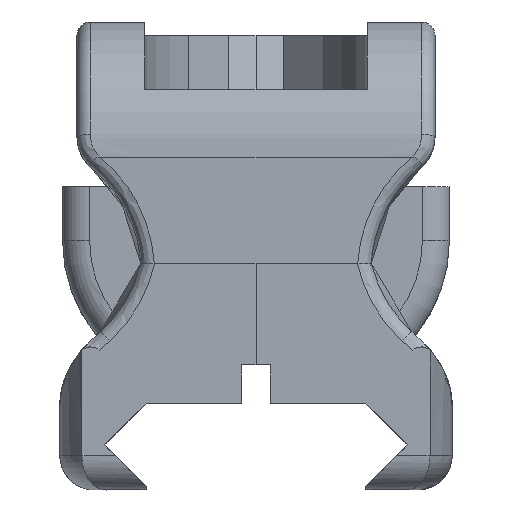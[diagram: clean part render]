
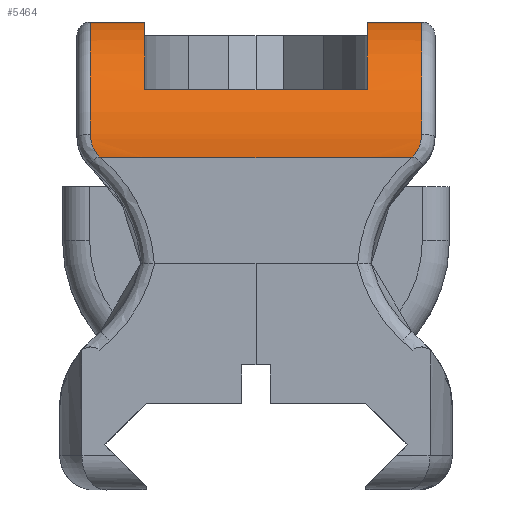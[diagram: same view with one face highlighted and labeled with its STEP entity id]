
A CAD part, front view. The second image highlights one B-rep face of the part: STEP entity #5464.
In plain terms, the highlighted cylindrical face has radius 10 mm (diameter 20 mm), a partial arc.
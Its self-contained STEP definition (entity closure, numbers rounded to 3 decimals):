
#151=B_SPLINE_CURVE_WITH_KNOTS('',3,(#8358,#8359,#8360,#8361,#8362),
 .UNSPECIFIED.,.F.,.F.,(4,1,4),(-0.17,-0.085,0.),
 .UNSPECIFIED.);
#167=B_SPLINE_CURVE_WITH_KNOTS('',3,(#8548,#8549,#8550,#8551,#8552,#8553,
#8554),.UNSPECIFIED.,.F.,.F.,(4,3,4),(-0.004,0.,0.005),
 .UNSPECIFIED.);
#248=B_SPLINE_CURVE_WITH_KNOTS('',3,(#10357,#10358,#10359,#10360,#10361),
 .UNSPECIFIED.,.F.,.F.,(4,1,4),(-0.17,-0.085,0.),
 .UNSPECIFIED.);
#260=B_SPLINE_CURVE_WITH_KNOTS('',3,(#10519,#10520,#10521,#10522,#10523,
#10524,#10525),.UNSPECIFIED.,.F.,.F.,(4,3,4),(-0.004,0.,0.005),
 .UNSPECIFIED.);
#382=CYLINDRICAL_SURFACE('',#5868,10.);
#394=CIRCLE('',#5491,10.);
#396=CIRCLE('',#5495,10.);
#431=CIRCLE('',#5583,10.);
#491=CIRCLE('',#5751,10.);
#522=CIRCLE('',#5866,10.);
#523=CIRCLE('',#5867,10.);
#809=FACE_OUTER_BOUND('',#1103,.T.);
#1103=EDGE_LOOP('',(#4987,#4988,#4989,#4990,#4991,#4992,#4993,#4994,#4995,
#4996,#4997,#4998,#4999,#5000,#5001,#5002));
#1115=LINE('',#7130,#1568);
#1243=LINE('',#8377,#1696);
#1424=LINE('',#10363,#1877);
#1554=LINE('',#11686,#2007);
#1555=LINE('',#11690,#2008);
#1556=LINE('',#11693,#2009);
#1568=VECTOR('',#5890,10.);
#1696=VECTOR('',#6220,10.);
#1877=VECTOR('',#6733,10.);
#2007=VECTOR('',#7089,10.);
#2008=VECTOR('',#7092,10.);
#2009=VECTOR('',#7095,10.);
#2021=VERTEX_POINT('',#7127);
#2022=VERTEX_POINT('',#7129);
#2042=VERTEX_POINT('',#7174);
#2046=VERTEX_POINT('',#7186);
#2208=VERTEX_POINT('',#8306);
#2209=VERTEX_POINT('',#8308);
#2211=VERTEX_POINT('',#8337);
#2226=VERTEX_POINT('',#8542);
#2415=VERTEX_POINT('',#10295);
#2416=VERTEX_POINT('',#10297);
#2418=VERTEX_POINT('',#10326);
#2432=VERTEX_POINT('',#10518);
#2538=VERTEX_POINT('',#11685);
#2539=VERTEX_POINT('',#11687);
#2540=VERTEX_POINT('',#11689);
#2541=VERTEX_POINT('',#11691);
#2552=EDGE_CURVE('',#2021,#2022,#1115,.T.);
#2576=EDGE_CURVE('',#2021,#2042,#394,.T.);
#2581=EDGE_CURVE('',#2022,#2046,#396,.T.);
#2789=EDGE_CURVE('',#2208,#2209,#431,.T.);
#2792=EDGE_CURVE('',#2211,#2208,#151,.T.);
#2797=EDGE_CURVE('',#2209,#2042,#1243,.T.);
#2816=EDGE_CURVE('',#2226,#2211,#167,.T.);
#3133=EDGE_CURVE('',#2415,#2416,#491,.T.);
#3137=EDGE_CURVE('',#2418,#2415,#248,.T.);
#3138=EDGE_CURVE('',#2416,#2046,#1424,.T.);
#3157=EDGE_CURVE('',#2432,#2418,#260,.T.);
#3361=EDGE_CURVE('',#2538,#2432,#1554,.T.);
#3362=EDGE_CURVE('',#2538,#2539,#522,.T.);
#3363=EDGE_CURVE('',#2539,#2540,#1555,.T.);
#3364=EDGE_CURVE('',#2541,#2540,#523,.T.);
#3365=EDGE_CURVE('',#2541,#2226,#1556,.T.);
#4987=ORIENTED_EDGE('',*,*,#3363,.F.);
#4988=ORIENTED_EDGE('',*,*,#3362,.F.);
#4989=ORIENTED_EDGE('',*,*,#3361,.T.);
#4990=ORIENTED_EDGE('',*,*,#3157,.T.);
#4991=ORIENTED_EDGE('',*,*,#3137,.T.);
#4992=ORIENTED_EDGE('',*,*,#3133,.T.);
#4993=ORIENTED_EDGE('',*,*,#3138,.T.);
#4994=ORIENTED_EDGE('',*,*,#2581,.F.);
#4995=ORIENTED_EDGE('',*,*,#2552,.F.);
#4996=ORIENTED_EDGE('',*,*,#2576,.T.);
#4997=ORIENTED_EDGE('',*,*,#2797,.F.);
#4998=ORIENTED_EDGE('',*,*,#2789,.F.);
#4999=ORIENTED_EDGE('',*,*,#2792,.F.);
#5000=ORIENTED_EDGE('',*,*,#2816,.F.);
#5001=ORIENTED_EDGE('',*,*,#3365,.F.);
#5002=ORIENTED_EDGE('',*,*,#3364,.T.);
#5464=ADVANCED_FACE('',(#809),#382,.T.);
#5491=AXIS2_PLACEMENT_3D('',#7176,#5921,#5922);
#5495=AXIS2_PLACEMENT_3D('',#7187,#5932,#5933);
#5583=AXIS2_PLACEMENT_3D('',#8309,#6211,#6212);
#5751=AXIS2_PLACEMENT_3D('',#10299,#6729,#6730);
#5866=AXIS2_PLACEMENT_3D('',#11688,#7090,#7091);
#5867=AXIS2_PLACEMENT_3D('',#11692,#7093,#7094);
#5868=AXIS2_PLACEMENT_3D('',#11694,#7096,#7097);
#5890=DIRECTION('',(1.,0.,0.));
#5921=DIRECTION('center_axis',(-1.,0.,0.));
#5922=DIRECTION('ref_axis',(0.,0.707,0.707));
#5932=DIRECTION('center_axis',(-1.,0.,
0.));
#5933=DIRECTION('ref_axis',(0.,0.707,0.707));
#6211=DIRECTION('center_axis',(-1.,0.,
0.));
#6212=DIRECTION('ref_axis',(0.,-0.804,0.595));
#6220=DIRECTION('',(1.,0.,0.));
#6729=DIRECTION('center_axis',(-1.,0.,
0.));
#6730=DIRECTION('ref_axis',(0.,-0.804,0.595));
#6733=DIRECTION('',(-1.,0.,0.));
#7089=DIRECTION('',(1.,0.,0.));
#7090=DIRECTION('center_axis',(1.,0.,0.));
#7091=DIRECTION('ref_axis',(0.,-0.707,0.707));
#7092=DIRECTION('',(-1.,0.,0.));
#7093=DIRECTION('center_axis',(1.,0.,0.));
#7094=DIRECTION('ref_axis',(0.,-0.707,0.707));
#7095=DIRECTION('',(-1.,0.,0.));
#7096=DIRECTION('center_axis',(-1.,0.,
0.));
#7097=DIRECTION('ref_axis',(0.,-0.707,0.707));
#7127=CARTESIAN_POINT('',(-8.185,-225.818,23.067));
#7129=CARTESIAN_POINT('',(8.237,-225.818,23.067));
#7130=CARTESIAN_POINT('',(-4.08,-225.818,23.067));
#7174=CARTESIAN_POINT('',(-8.185,-217.221,28.066));
#7176=CARTESIAN_POINT('Origin',(-8.185,-217.157,18.067));
#7186=CARTESIAN_POINT('',(8.237,-217.221,28.066));
#7187=CARTESIAN_POINT('Origin',(8.237,-217.157,18.067));
#8306=CARTESIAN_POINT('',(-12.185,-227.011,19.769));
#8308=CARTESIAN_POINT('',(-12.185,-217.221,28.066));
#8309=CARTESIAN_POINT('Origin',(-12.185,-217.157,18.067));
#8337=CARTESIAN_POINT('',(-11.513,-227.157,18.108));
#8358=CARTESIAN_POINT('Ctrl Pts',(-11.513,-227.157,18.108));
#8359=CARTESIAN_POINT('Ctrl Pts',(-11.725,-227.156,18.316));
#8360=CARTESIAN_POINT('Ctrl Pts',(-12.067,-227.141,18.835));
#8361=CARTESIAN_POINT('Ctrl Pts',(-12.185,-227.065,19.46));
#8362=CARTESIAN_POINT('Ctrl Pts',(-12.185,-227.011,19.769));
#8377=CARTESIAN_POINT('',(4.131,-217.221,28.066));
#8542=CARTESIAN_POINT('',(-11.443,-227.157,18.067));
#8548=CARTESIAN_POINT('Ctrl Pts',(-11.443,-227.157,18.067));
#8549=CARTESIAN_POINT('Ctrl Pts',(-11.453,-227.157,18.073));
#8550=CARTESIAN_POINT('Ctrl Pts',(-11.464,-227.157,18.079));
#8551=CARTESIAN_POINT('Ctrl Pts',(-11.474,-227.157,18.085));
#8552=CARTESIAN_POINT('Ctrl Pts',(-11.487,-227.157,18.092));
#8553=CARTESIAN_POINT('Ctrl Pts',(-11.5,-227.157,18.1));
#8554=CARTESIAN_POINT('Ctrl Pts',(-11.513,-227.157,18.108));
#10295=CARTESIAN_POINT('',(12.237,-227.011,19.769));
#10297=CARTESIAN_POINT('',(12.237,-217.221,28.066));
#10299=CARTESIAN_POINT('Origin',(12.237,-217.157,18.067));
#10326=CARTESIAN_POINT('',(11.565,-227.157,18.108));
#10357=CARTESIAN_POINT('Ctrl Pts',(11.565,-227.157,18.108));
#10358=CARTESIAN_POINT('Ctrl Pts',(11.776,-227.156,18.316));
#10359=CARTESIAN_POINT('Ctrl Pts',(12.118,-227.141,18.835));
#10360=CARTESIAN_POINT('Ctrl Pts',(12.237,-227.065,19.46));
#10361=CARTESIAN_POINT('Ctrl Pts',(12.237,-227.011,19.769));
#10363=CARTESIAN_POINT('',(-4.08,-217.221,28.066));
#10518=CARTESIAN_POINT('',(11.494,-227.157,18.067));
#10519=CARTESIAN_POINT('Ctrl Pts',(11.494,-227.157,18.067));
#10520=CARTESIAN_POINT('Ctrl Pts',(11.505,-227.157,18.073));
#10521=CARTESIAN_POINT('Ctrl Pts',(11.515,-227.157,18.079));
#10522=CARTESIAN_POINT('Ctrl Pts',(11.525,-227.157,18.085));
#10523=CARTESIAN_POINT('Ctrl Pts',(11.538,-227.157,18.092));
#10524=CARTESIAN_POINT('Ctrl Pts',(11.552,-227.157,18.1));
#10525=CARTESIAN_POINT('Ctrl Pts',(11.565,-227.157,18.108));
#11685=CARTESIAN_POINT('',(8.237,-227.157,18.067));
#11686=CARTESIAN_POINT('',(8.237,-227.157,18.067));
#11687=CARTESIAN_POINT('',(8.237,-227.157,18.066));
#11688=CARTESIAN_POINT('Origin',(8.237,-217.157,18.067));
#11689=CARTESIAN_POINT('',(-8.185,-227.157,18.066));
#11690=CARTESIAN_POINT('',(-4.08,-227.157,18.066));
#11691=CARTESIAN_POINT('',(-8.185,-227.157,18.067));
#11692=CARTESIAN_POINT('Origin',(-8.185,-217.157,18.067));
#11693=CARTESIAN_POINT('',(-8.185,-227.157,18.067));
#11694=CARTESIAN_POINT('Origin',(4.131,-217.157,18.067));
